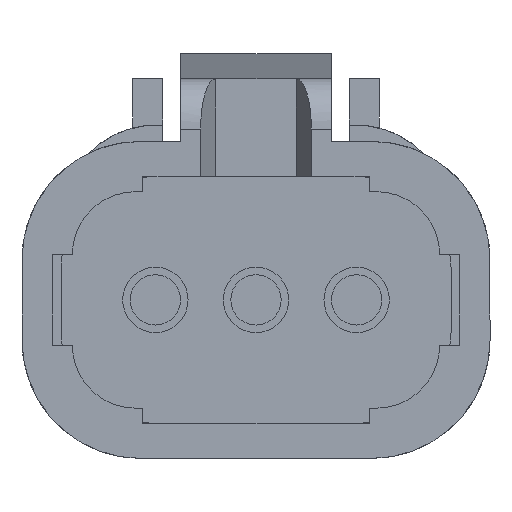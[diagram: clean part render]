
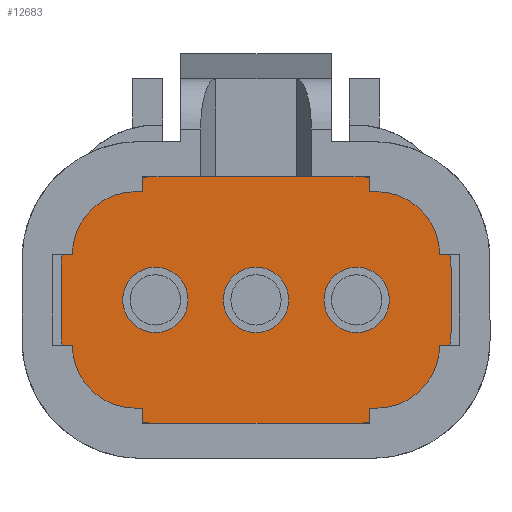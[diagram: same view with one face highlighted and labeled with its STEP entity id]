
A CAD part, front view. The second image highlights one B-rep face of the part: STEP entity #12683.
In plain terms, the highlighted planar face has unit normal (0, -1, 0).
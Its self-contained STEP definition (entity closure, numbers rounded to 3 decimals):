
#6 = ORIENTED_EDGE ( 'NONE', *, *, #4839, .F. ) ;
#62 = EDGE_CURVE ( 'NONE', #1201, #10779, #12657, .T. ) ;
#114 = DIRECTION ( 'NONE',  ( 1., 0., 0. ) ) ;
#271 = VECTOR ( 'NONE', #5045, 1000. ) ;
#339 = CARTESIAN_POINT ( 'NONE',  ( 5.634, 3.703, 12.772 ) ) ;
#397 = CARTESIAN_POINT ( 'NONE',  ( 3.559, 3.703, 10.322 ) ) ;
#438 = CARTESIAN_POINT ( 'NONE',  ( 1.484, 3.703, 9.672 ) ) ;
#455 = CARTESIAN_POINT ( 'NONE',  ( 4.909, 3.703, 10.322 ) ) ;
#548 = DIRECTION ( 'NONE',  ( 0., -1., 0. ) ) ;
#696 = CIRCLE ( 'NONE', #4889, 0.65 ) ;
#788 = EDGE_LOOP ( 'NONE', ( #7591, #8454 ) ) ;
#876 = DIRECTION ( 'NONE',  ( 1., 0., 0. ) ) ;
#936 = DIRECTION ( 'NONE',  ( 0., 1., 0. ) ) ;
#941 = VECTOR ( 'NONE', #7160, 1000. ) ;
#1018 = CIRCLE ( 'NONE', #12538, 0.65 ) ;
#1055 = EDGE_CURVE ( 'NONE', #3977, #6118, #1140, .T. ) ;
#1140 = LINE ( 'NONE', #3969, #941 ) ;
#1161 = CARTESIAN_POINT ( 'NONE',  ( 2.209, 3.703, 10.322 ) ) ;
#1201 = VERTEX_POINT ( 'NONE', #1332 ) ;
#1332 = CARTESIAN_POINT ( 'NONE',  ( 0.909, 3.703, 10.322 ) ) ;
#1480 = DIRECTION ( 'NONE',  ( -1., 0., 0. ) ) ;
#1521 = CIRCLE ( 'NONE', #6313, 1.8 ) ;
#1635 = ORIENTED_EDGE ( 'NONE', *, *, #4170, .F. ) ;
#1875 = FACE_BOUND ( 'NONE', #788, .T. ) ;
#1933 = EDGE_LOOP ( 'NONE', ( #7578, #3388, #6548, #10974, #8785, #11515, #6, #1635 ) ) ;
#2562 = VERTEX_POINT ( 'NONE', #6940 ) ;
#2833 = CARTESIAN_POINT ( 'NONE',  ( 1.484, 3.703, 7.872 ) ) ;
#2983 = DIRECTION ( 'NONE',  ( 0., -1., 0. ) ) ;
#3377 = VECTOR ( 'NONE', #10843, 1000. ) ;
#3388 = ORIENTED_EDGE ( 'NONE', *, *, #1055, .F. ) ;
#3593 = VERTEX_POINT ( 'NONE', #9386 ) ;
#3790 = CARTESIAN_POINT ( 'NONE',  ( 5.559, 3.703, 10.322 ) ) ;
#3869 = CARTESIAN_POINT ( 'NONE',  ( 6.209, 3.703, 10.322 ) ) ;
#3872 = LINE ( 'NONE', #7851, #7261 ) ;
#3876 = CIRCLE ( 'NONE', #8039, 0.65 ) ;
#3969 = CARTESIAN_POINT ( 'NONE',  ( 5.634, 3.703, 7.872 ) ) ;
#3977 = VERTEX_POINT ( 'NONE', #5123 ) ;
#4032 = DIRECTION ( 'NONE',  ( -1., 0., 0. ) ) ;
#4034 = CARTESIAN_POINT ( 'NONE',  ( -0.316, 3.703, 10.972 ) ) ;
#4104 = CIRCLE ( 'NONE', #7864, 0.65 ) ;
#4108 = AXIS2_PLACEMENT_3D ( 'NONE', #7795, #11794, #7857 ) ;
#4170 = EDGE_CURVE ( 'NONE', #9308, #4676, #12859, .T. ) ;
#4658 = ORIENTED_EDGE ( 'NONE', *, *, #8499, .F. ) ;
#4676 = VERTEX_POINT ( 'NONE', #4034 ) ;
#4741 = AXIS2_PLACEMENT_3D ( 'NONE', #10373, #6180, #1480 ) ;
#4800 = ORIENTED_EDGE ( 'NONE', *, *, #11063, .F. ) ;
#4839 = EDGE_CURVE ( 'NONE', #4676, #12501, #6004, .T. ) ;
#4889 = AXIS2_PLACEMENT_3D ( 'NONE', #8654, #7738, #10814 ) ;
#4899 = CARTESIAN_POINT ( 'NONE',  ( 2.909, 3.703, 10.322 ) ) ;
#4937 = DIRECTION ( 'NONE',  ( 0., -1., 0. ) ) ;
#5045 = DIRECTION ( 'NONE',  ( 0., 0., 1. ) ) ;
#5123 = CARTESIAN_POINT ( 'NONE',  ( 5.634, 3.703, 7.872 ) ) ;
#5281 = CARTESIAN_POINT ( 'NONE',  ( 1.484, 3.703, 12.772 ) ) ;
#5308 = CARTESIAN_POINT ( 'NONE',  ( 7.434, 3.703, 10.972 ) ) ;
#5659 = CARTESIAN_POINT ( 'NONE',  ( 5.559, 3.703, 10.322 ) ) ;
#5882 = EDGE_CURVE ( 'NONE', #9410, #2562, #12280, .T. ) ;
#6004 = CIRCLE ( 'NONE', #4741, 1.8 ) ;
#6118 = VERTEX_POINT ( 'NONE', #2833 ) ;
#6180 = DIRECTION ( 'NONE',  ( 0., 1., 0. ) ) ;
#6313 = AXIS2_PLACEMENT_3D ( 'NONE', #7339, #8325, #10425 ) ;
#6548 = ORIENTED_EDGE ( 'NONE', *, *, #7194, .F. ) ;
#6634 = AXIS2_PLACEMENT_3D ( 'NONE', #397, #8322, #11274 ) ;
#6820 = CARTESIAN_POINT ( 'NONE',  ( -0.316, 3.703, 9.672 ) ) ;
#6896 = CARTESIAN_POINT ( 'NONE',  ( 3.559, 3.703, 10.322 ) ) ;
#6913 = AXIS2_PLACEMENT_3D ( 'NONE', #10802, #9887, #114 ) ;
#6940 = CARTESIAN_POINT ( 'NONE',  ( 4.209, 3.703, 10.322 ) ) ;
#6955 = CARTESIAN_POINT ( 'NONE',  ( 1.484, 3.703, 9.672 ) ) ;
#7129 = VERTEX_POINT ( 'NONE', #339 ) ;
#7160 = DIRECTION ( 'NONE',  ( -1., 0., 0. ) ) ;
#7194 = EDGE_CURVE ( 'NONE', #3593, #3977, #1521, .T. ) ;
#7261 = VECTOR ( 'NONE', #10992, 1000. ) ;
#7339 = CARTESIAN_POINT ( 'NONE',  ( 5.634, 3.703, 9.672 ) ) ;
#7578 = ORIENTED_EDGE ( 'NONE', *, *, #8020, .F. ) ;
#7591 = ORIENTED_EDGE ( 'NONE', *, *, #62, .F. ) ;
#7738 = DIRECTION ( 'NONE',  ( 0., -1., 0. ) ) ;
#7795 = CARTESIAN_POINT ( 'NONE',  ( 1.559, 3.703, 10.322 ) ) ;
#7838 = EDGE_CURVE ( 'NONE', #10528, #3593, #3872, .T. ) ;
#7851 = CARTESIAN_POINT ( 'NONE',  ( 7.434, 3.703, 9.672 ) ) ;
#7857 = DIRECTION ( 'NONE',  ( -1., 0., 0. ) ) ;
#7864 = AXIS2_PLACEMENT_3D ( 'NONE', #3790, #2983, #4032 ) ;
#8020 = EDGE_CURVE ( 'NONE', #6118, #9308, #10416, .T. ) ;
#8039 = AXIS2_PLACEMENT_3D ( 'NONE', #6896, #4937, #11945 ) ;
#8128 = AXIS2_PLACEMENT_3D ( 'NONE', #438, #11653, #8696 ) ;
#8314 = EDGE_LOOP ( 'NONE', ( #4658, #4800 ) ) ;
#8322 = DIRECTION ( 'NONE',  ( 0., -1., 0. ) ) ;
#8325 = DIRECTION ( 'NONE',  ( 0., 1., 0. ) ) ;
#8454 = ORIENTED_EDGE ( 'NONE', *, *, #11810, .F. ) ;
#8499 = EDGE_CURVE ( 'NONE', #10561, #12246, #1018, .T. ) ;
#8538 = DIRECTION ( 'NONE',  ( -1., 0., 0. ) ) ;
#8654 = CARTESIAN_POINT ( 'NONE',  ( 1.559, 3.703, 10.322 ) ) ;
#8696 = DIRECTION ( 'NONE',  ( 1., 0., 0. ) ) ;
#8785 = ORIENTED_EDGE ( 'NONE', *, *, #8914, .F. ) ;
#8914 = EDGE_CURVE ( 'NONE', #7129, #10528, #10043, .T. ) ;
#8982 = FACE_OUTER_BOUND ( 'NONE', #1933, .T. ) ;
#9308 = VERTEX_POINT ( 'NONE', #9614 ) ;
#9386 = CARTESIAN_POINT ( 'NONE',  ( 7.434, 3.703, 9.672 ) ) ;
#9410 = VERTEX_POINT ( 'NONE', #4899 ) ;
#9506 = ORIENTED_EDGE ( 'NONE', *, *, #12694, .F. ) ;
#9614 = CARTESIAN_POINT ( 'NONE',  ( -0.316, 3.703, 9.672 ) ) ;
#9793 = EDGE_CURVE ( 'NONE', #12501, #7129, #12755, .T. ) ;
#9848 = PLANE ( 'NONE',  #12867 ) ;
#9887 = DIRECTION ( 'NONE',  ( 0., 1., 0. ) ) ;
#10043 = CIRCLE ( 'NONE', #6913, 1.8 ) ;
#10185 = EDGE_LOOP ( 'NONE', ( #12952, #9506 ) ) ;
#10373 = CARTESIAN_POINT ( 'NONE',  ( 1.484, 3.703, 10.972 ) ) ;
#10416 = CIRCLE ( 'NONE', #8128, 1.8 ) ;
#10425 = DIRECTION ( 'NONE',  ( -1., 0., 0. ) ) ;
#10528 = VERTEX_POINT ( 'NONE', #5308 ) ;
#10561 = VERTEX_POINT ( 'NONE', #455 ) ;
#10779 = VERTEX_POINT ( 'NONE', #1161 ) ;
#10802 = CARTESIAN_POINT ( 'NONE',  ( 5.634, 3.703, 10.972 ) ) ;
#10814 = DIRECTION ( 'NONE',  ( -1., 0., 0. ) ) ;
#10843 = DIRECTION ( 'NONE',  ( 1., 0., 0. ) ) ;
#10974 = ORIENTED_EDGE ( 'NONE', *, *, #7838, .F. ) ;
#10992 = DIRECTION ( 'NONE',  ( 0., 0., -1. ) ) ;
#11063 = EDGE_CURVE ( 'NONE', #12246, #10561, #4104, .T. ) ;
#11274 = DIRECTION ( 'NONE',  ( -1., 0., 0. ) ) ;
#11515 = ORIENTED_EDGE ( 'NONE', *, *, #9793, .F. ) ;
#11653 = DIRECTION ( 'NONE',  ( 0., 1., 0. ) ) ;
#11794 = DIRECTION ( 'NONE',  ( 0., -1., 0. ) ) ;
#11810 = EDGE_CURVE ( 'NONE', #10779, #1201, #696, .T. ) ;
#11828 = CARTESIAN_POINT ( 'NONE',  ( 5.634, 3.703, 12.772 ) ) ;
#11885 = FACE_BOUND ( 'NONE', #8314, .T. ) ;
#11945 = DIRECTION ( 'NONE',  ( -1., 0., 0. ) ) ;
#12246 = VERTEX_POINT ( 'NONE', #3869 ) ;
#12280 = CIRCLE ( 'NONE', #6634, 0.65 ) ;
#12501 = VERTEX_POINT ( 'NONE', #5281 ) ;
#12538 = AXIS2_PLACEMENT_3D ( 'NONE', #5659, #548, #8538 ) ;
#12657 = CIRCLE ( 'NONE', #4108, 0.65 ) ;
#12683 = ADVANCED_FACE ( 'NONE', ( #1875, #12873, #11885, #8982 ), #9848, .F. ) ;
#12694 = EDGE_CURVE ( 'NONE', #2562, #9410, #3876, .T. ) ;
#12755 = LINE ( 'NONE', #11828, #3377 ) ;
#12859 = LINE ( 'NONE', #6820, #271 ) ;
#12867 = AXIS2_PLACEMENT_3D ( 'NONE', #6955, #936, #876 ) ;
#12873 = FACE_BOUND ( 'NONE', #10185, .T. ) ;
#12952 = ORIENTED_EDGE ( 'NONE', *, *, #5882, .F. ) ;
